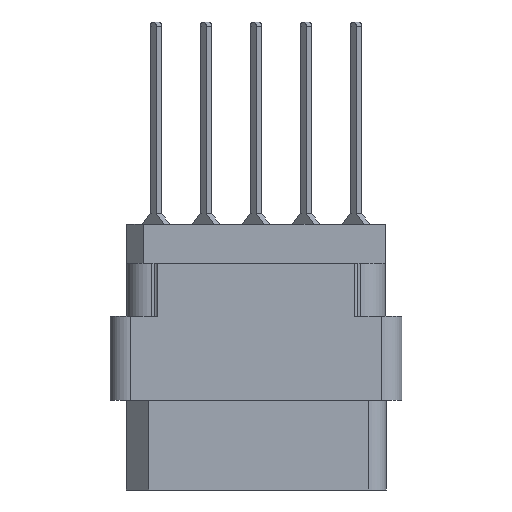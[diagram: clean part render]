
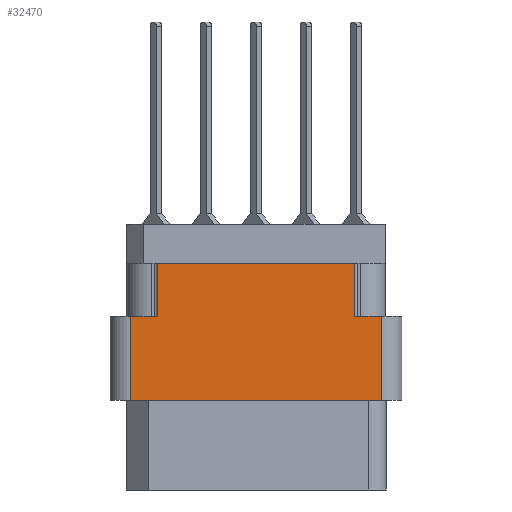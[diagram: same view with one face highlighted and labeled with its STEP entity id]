
A CAD part, left-side view. The second image highlights one B-rep face of the part: STEP entity #32470.
In plain terms, the highlighted planar face has unit normal (-1, 0, 0).
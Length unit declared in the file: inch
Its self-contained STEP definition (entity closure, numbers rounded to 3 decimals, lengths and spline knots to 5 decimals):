
#499 = VECTOR ( 'NONE', #21133, 39.37008 ) ;
#519 = LINE ( 'NONE', #708, #4650 ) ;
#527 = CARTESIAN_POINT ( 'NONE',  ( -1., 0.438, -0.277 ) ) ;
#708 = CARTESIAN_POINT ( 'NONE',  ( -1., -0.376, -0.798 ) ) ;
#1116 = VERTEX_POINT ( 'NONE', #24646 ) ;
#1919 = VECTOR ( 'NONE', #21616, 39.37008 ) ;
#2419 = VERTEX_POINT ( 'NONE', #15651 ) ;
#3264 = CARTESIAN_POINT ( 'NONE',  ( -1., -0.376, -0.798 ) ) ;
#4527 = VECTOR ( 'NONE', #24255, 39.37008 ) ;
#4650 = VECTOR ( 'NONE', #6572, 39.37008 ) ;
#4866 = CARTESIAN_POINT ( 'NONE',  ( -1., 0.376, -0.798 ) ) ;
#5902 = EDGE_CURVE ( 'NONE', #9651, #27240, #21320, .T. ) ;
#6572 = DIRECTION ( 'NONE',  ( 0., 0., 1. ) ) ;
#7092 = ORIENTED_EDGE ( 'NONE', *, *, #12131, .F. ) ;
#9616 = EDGE_LOOP ( 'NONE', ( #24838, #19767, #18125, #9773, #13436, #25265, #7092, #31624 ) ) ;
#9651 = VERTEX_POINT ( 'NONE', #17515 ) ;
#9773 = ORIENTED_EDGE ( 'NONE', *, *, #16011, .F. ) ;
#10386 = LINE ( 'NONE', #4866, #1919 ) ;
#11263 = AXIS2_PLACEMENT_3D ( 'NONE', #3264, #26264, #14667 ) ;
#11904 = PLANE ( 'NONE',  #11263 ) ;
#12131 = EDGE_CURVE ( 'NONE', #14410, #19797, #21695, .T. ) ;
#12872 = EDGE_CURVE ( 'NONE', #15754, #1116, #519, .T. ) ;
#13034 = CARTESIAN_POINT ( 'NONE',  ( -1., 0.296, -0.277 ) ) ;
#13415 = DIRECTION ( 'NONE',  ( 0., -1., 0. ) ) ;
#13436 = ORIENTED_EDGE ( 'NONE', *, *, #5902, .T. ) ;
#14410 = VERTEX_POINT ( 'NONE', #15480 ) ;
#14667 = DIRECTION ( 'NONE',  ( 0., 0., 1. ) ) ;
#14859 = LINE ( 'NONE', #527, #31966 ) ;
#15213 = EDGE_CURVE ( 'NONE', #25772, #14410, #14859, .T. ) ;
#15480 = CARTESIAN_POINT ( 'NONE',  ( -1., 0.296, -0.277 ) ) ;
#15651 = CARTESIAN_POINT ( 'NONE',  ( -1., 0.376, -0.529 ) ) ;
#15754 = VERTEX_POINT ( 'NONE', #21267 ) ;
#15989 = CARTESIAN_POINT ( 'NONE',  ( -1., -0.296, -0.117 ) ) ;
#16011 = EDGE_CURVE ( 'NONE', #9651, #1116, #27549, .T. ) ;
#16718 = CARTESIAN_POINT ( 'NONE',  ( -1., 0.438, -0.117 ) ) ;
#17515 = CARTESIAN_POINT ( 'NONE',  ( -1., -0.296, -0.277 ) ) ;
#17967 = VECTOR ( 'NONE', #13415, 39.37008 ) ;
#18125 = ORIENTED_EDGE ( 'NONE', *, *, #12872, .T. ) ;
#18955 = DIRECTION ( 'NONE',  ( 0., 1., 0. ) ) ;
#19266 = DIRECTION ( 'NONE',  ( 0., -1., 0. ) ) ;
#19767 = ORIENTED_EDGE ( 'NONE', *, *, #25446, .F. ) ;
#19797 = VERTEX_POINT ( 'NONE', #20711 ) ;
#20711 = CARTESIAN_POINT ( 'NONE',  ( -1., 0.296, -0.117 ) ) ;
#21133 = DIRECTION ( 'NONE',  ( 0., 0., 1. ) ) ;
#21185 = LINE ( 'NONE', #32932, #21585 ) ;
#21267 = CARTESIAN_POINT ( 'NONE',  ( -1., -0.376, -0.529 ) ) ;
#21320 = LINE ( 'NONE', #27195, #499 ) ;
#21585 = VECTOR ( 'NONE', #18955, 39.37008 ) ;
#21616 = DIRECTION ( 'NONE',  ( 0., 0., 1. ) ) ;
#21695 = LINE ( 'NONE', #13034, #4527 ) ;
#22232 = EDGE_CURVE ( 'NONE', #19797, #27240, #32916, .T. ) ;
#24255 = DIRECTION ( 'NONE',  ( 0., 0., 1. ) ) ;
#24646 = CARTESIAN_POINT ( 'NONE',  ( -1., -0.376, -0.277 ) ) ;
#24838 = ORIENTED_EDGE ( 'NONE', *, *, #33318, .F. ) ;
#25265 = ORIENTED_EDGE ( 'NONE', *, *, #22232, .F. ) ;
#25446 = EDGE_CURVE ( 'NONE', #15754, #2419, #21185, .T. ) ;
#25772 = VERTEX_POINT ( 'NONE', #35476 ) ;
#26264 = DIRECTION ( 'NONE',  ( -1., 0., 0. ) ) ;
#27195 = CARTESIAN_POINT ( 'NONE',  ( -1., -0.296, -0.277 ) ) ;
#27240 = VERTEX_POINT ( 'NONE', #15989 ) ;
#27549 = LINE ( 'NONE', #33605, #32568 ) ;
#31624 = ORIENTED_EDGE ( 'NONE', *, *, #15213, .F. ) ;
#31966 = VECTOR ( 'NONE', #34533, 39.37008 ) ;
#32470 = ADVANCED_FACE ( 'NONE', ( #36015 ), #11904, .T. ) ;
#32568 = VECTOR ( 'NONE', #19266, 39.37008 ) ;
#32916 = LINE ( 'NONE', #16718, #17967 ) ;
#32932 = CARTESIAN_POINT ( 'NONE',  ( -1., -0.376, -0.529 ) ) ;
#33318 = EDGE_CURVE ( 'NONE', #2419, #25772, #10386, .T. ) ;
#33605 = CARTESIAN_POINT ( 'NONE',  ( -1., -0.296, -0.277 ) ) ;
#34533 = DIRECTION ( 'NONE',  ( 0., -1., 0. ) ) ;
#35476 = CARTESIAN_POINT ( 'NONE',  ( -1., 0.376, -0.277 ) ) ;
#36015 = FACE_OUTER_BOUND ( 'NONE', #9616, .T. ) ;
